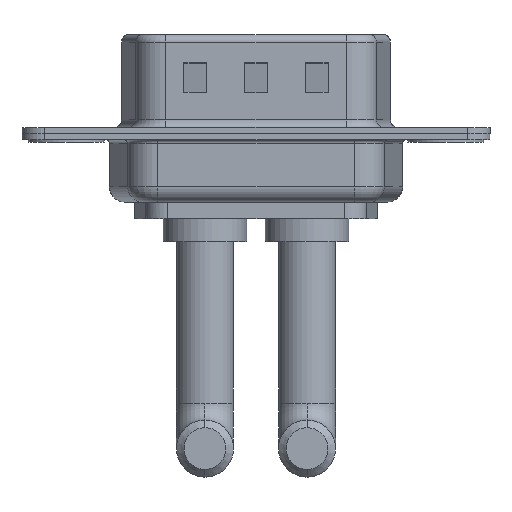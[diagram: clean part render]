
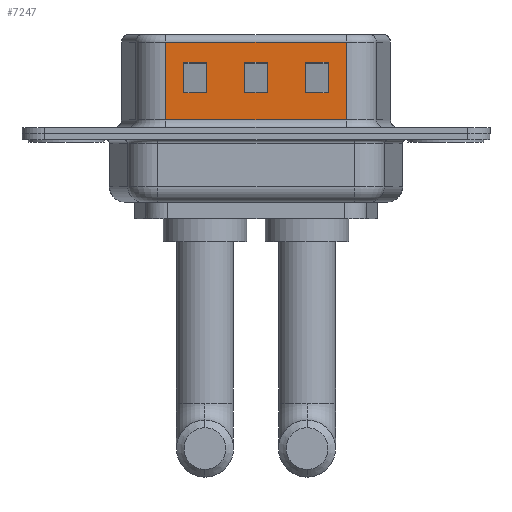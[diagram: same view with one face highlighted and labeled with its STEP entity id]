
A CAD part, front view. The second image highlights one B-rep face of the part: STEP entity #7247.
In plain terms, the highlighted planar face has unit normal (0, -1, 0).
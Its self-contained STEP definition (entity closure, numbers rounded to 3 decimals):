
#144 = CARTESIAN_POINT ( 'NONE',  ( 17.25, -4.55, 4.705 ) ) ;
#253 = VERTEX_POINT ( 'NONE', #11063 ) ;
#267 = VECTOR ( 'NONE', #5261, 1000. ) ;
#295 = EDGE_CURVE ( 'NONE', #964, #10683, #6149, .T. ) ;
#341 = DIRECTION ( 'NONE',  ( 0., 1., 0. ) ) ;
#506 = CARTESIAN_POINT ( 'NONE',  ( 6.549, -4.55, 6.52 ) ) ;
#653 = VECTOR ( 'NONE', #3412, 1000. ) ;
#688 = VECTOR ( 'NONE', #11170, 1000. ) ;
#964 = VERTEX_POINT ( 'NONE', #9049 ) ;
#1160 = EDGE_CURVE ( 'NONE', #10683, #10582, #6900, .T. ) ;
#1284 = DIRECTION ( 'NONE',  ( -1., 0., 0. ) ) ;
#1363 = CARTESIAN_POINT ( 'NONE',  ( 14.451, -4.55, 4.705 ) ) ;
#1442 = ORIENTED_EDGE ( 'NONE', *, *, #1997, .T. ) ;
#1643 = VECTOR ( 'NONE', #6165, 1000. ) ;
#1785 = CARTESIAN_POINT ( 'NONE',  ( 6.549, -4.55, 6.02 ) ) ;
#1997 = EDGE_CURVE ( 'NONE', #6853, #8826, #4202, .T. ) ;
#2039 = CARTESIAN_POINT ( 'NONE',  ( 13.25, -4.55, 2.705 ) ) ;
#2071 = EDGE_CURVE ( 'NONE', #9340, #253, #3422, .T. ) ;
#2237 = FACE_BOUND ( 'NONE', #9575, .T. ) ;
#2281 = EDGE_LOOP ( 'NONE', ( #9515, #8739, #8007, #7987 ) ) ;
#2312 = ORIENTED_EDGE ( 'NONE', *, *, #5085, .T. ) ;
#2397 = CARTESIAN_POINT ( 'NONE',  ( 9.25, -4.55, 6.52 ) ) ;
#2777 = VECTOR ( 'NONE', #11367, 1000. ) ;
#2842 = EDGE_CURVE ( 'NONE', #8517, #9124, #3017, .T. ) ;
#2870 = VECTOR ( 'NONE', #12316, 1000. ) ;
#3017 = LINE ( 'NONE', #1363, #4878 ) ;
#3307 = VECTOR ( 'NONE', #10962, 1000. ) ;
#3375 = VERTEX_POINT ( 'NONE', #144 ) ;
#3412 = DIRECTION ( 'NONE',  ( -1., 0., 0. ) ) ;
#3422 = LINE ( 'NONE', #7482, #2777 ) ;
#3617 = CARTESIAN_POINT ( 'NONE',  ( 13.25, -4.55, 4.705 ) ) ;
#3767 = ORIENTED_EDGE ( 'NONE', *, *, #3892, .T. ) ;
#3892 = EDGE_CURVE ( 'NONE', #3948, #8653, #11159, .T. ) ;
#3900 = LINE ( 'NONE', #7791, #11206 ) ;
#3910 = VECTOR ( 'NONE', #8266, 1000. ) ;
#3948 = VERTEX_POINT ( 'NONE', #9198 ) ;
#4017 = CARTESIAN_POINT ( 'NONE',  ( 17.25, -4.55, 6.52 ) ) ;
#4044 = DIRECTION ( 'NONE',  ( 0., 0., 1. ) ) ;
#4202 = LINE ( 'NONE', #6280, #1643 ) ;
#4217 = FACE_BOUND ( 'NONE', #6305, .T. ) ;
#4375 = ORIENTED_EDGE ( 'NONE', *, *, #2842, .T. ) ;
#4878 = VECTOR ( 'NONE', #10030, 1000. ) ;
#5085 = EDGE_CURVE ( 'NONE', #5225, #9340, #10999, .T. ) ;
#5095 = CARTESIAN_POINT ( 'NONE',  ( 18.451, -4.55, 2.705 ) ) ;
#5136 = DIRECTION ( 'NONE',  ( 0., 0., -1. ) ) ;
#5143 = VECTOR ( 'NONE', #4044, 1000. ) ;
#5175 = FACE_OUTER_BOUND ( 'NONE', #9629, .T. ) ;
#5225 = VERTEX_POINT ( 'NONE', #1785 ) ;
#5229 = DIRECTION ( 'NONE',  ( 0., 0., -1. ) ) ;
#5239 = ORIENTED_EDGE ( 'NONE', *, *, #6172, .T. ) ;
#5261 = DIRECTION ( 'NONE',  ( 0., 0., 1. ) ) ;
#5322 = CARTESIAN_POINT ( 'NONE',  ( 18.451, -4.55, 6.02 ) ) ;
#5388 = ORIENTED_EDGE ( 'NONE', *, *, #11726, .F. ) ;
#5398 = DIRECTION ( 'NONE',  ( 1., 0., 0. ) ) ;
#5462 = ORIENTED_EDGE ( 'NONE', *, *, #12061, .T. ) ;
#5811 = CARTESIAN_POINT ( 'NONE',  ( 9.25, -4.55, 4.705 ) ) ;
#5989 = LINE ( 'NONE', #4017, #10405 ) ;
#6106 = PLANE ( 'NONE',  #8422 ) ;
#6149 = LINE ( 'NONE', #7097, #653 ) ;
#6165 = DIRECTION ( 'NONE',  ( -1., 0., 0. ) ) ;
#6172 = EDGE_CURVE ( 'NONE', #12461, #10830, #7255, .T. ) ;
#6252 = LINE ( 'NONE', #12365, #10205 ) ;
#6280 = CARTESIAN_POINT ( 'NONE',  ( 14.451, -4.55, 2.705 ) ) ;
#6305 = EDGE_LOOP ( 'NONE', ( #3767, #5462, #5239, #12382 ) ) ;
#6853 = VERTEX_POINT ( 'NONE', #7168 ) ;
#6900 = LINE ( 'NONE', #9080, #5143 ) ;
#7043 = CARTESIAN_POINT ( 'NONE',  ( 11.75, -4.55, 2.705 ) ) ;
#7054 = EDGE_CURVE ( 'NONE', #9056, #5225, #7284, .T. ) ;
#7097 = CARTESIAN_POINT ( 'NONE',  ( 22.451, -4.55, 2.705 ) ) ;
#7168 = CARTESIAN_POINT ( 'NONE',  ( 9.25, -4.55, 2.705 ) ) ;
#7247 = ADVANCED_FACE ( 'NONE', ( #2237, #9059, #4217, #5175 ), #6106, .F. ) ;
#7255 = LINE ( 'NONE', #5095, #11838 ) ;
#7284 = LINE ( 'NONE', #5322, #688 ) ;
#7341 = ORIENTED_EDGE ( 'NONE', *, *, #12446, .T. ) ;
#7358 = CARTESIAN_POINT ( 'NONE',  ( 22.451, -4.55, 4.705 ) ) ;
#7482 = CARTESIAN_POINT ( 'NONE',  ( 18.451, -4.55, 0.9 ) ) ;
#7503 = VECTOR ( 'NONE', #5136, 1000. ) ;
#7791 = CARTESIAN_POINT ( 'NONE',  ( 11.75, -4.55, 6.52 ) ) ;
#7889 = LINE ( 'NONE', #11766, #267 ) ;
#7987 = ORIENTED_EDGE ( 'NONE', *, *, #11320, .T. ) ;
#8007 = ORIENTED_EDGE ( 'NONE', *, *, #1160, .T. ) ;
#8093 = CARTESIAN_POINT ( 'NONE',  ( 18.451, -4.55, 6.52 ) ) ;
#8266 = DIRECTION ( 'NONE',  ( 0., 0., -1. ) ) ;
#8272 = CARTESIAN_POINT ( 'NONE',  ( 15.75, -4.55, 4.705 ) ) ;
#8422 = AXIS2_PLACEMENT_3D ( 'NONE', #8093, #341, #11966 ) ;
#8429 = DIRECTION ( 'NONE',  ( 0., 0., -1. ) ) ;
#8430 = CARTESIAN_POINT ( 'NONE',  ( 18.451, -4.55, 4.705 ) ) ;
#8455 = CARTESIAN_POINT ( 'NONE',  ( 15.75, -4.55, 2.705 ) ) ;
#8517 = VERTEX_POINT ( 'NONE', #10324 ) ;
#8653 = VERTEX_POINT ( 'NONE', #3617 ) ;
#8739 = ORIENTED_EDGE ( 'NONE', *, *, #295, .T. ) ;
#8772 = ORIENTED_EDGE ( 'NONE', *, *, #8790, .T. ) ;
#8790 = EDGE_CURVE ( 'NONE', #9124, #6853, #10870, .T. ) ;
#8826 = VERTEX_POINT ( 'NONE', #11934 ) ;
#8997 = LINE ( 'NONE', #9837, #3307 ) ;
#9049 = CARTESIAN_POINT ( 'NONE',  ( 17.25, -4.55, 2.705 ) ) ;
#9056 = VERTEX_POINT ( 'NONE', #10480 ) ;
#9059 = FACE_BOUND ( 'NONE', #2281, .T. ) ;
#9080 = CARTESIAN_POINT ( 'NONE',  ( 15.75, -4.55, 6.52 ) ) ;
#9096 = CARTESIAN_POINT ( 'NONE',  ( 6.549, -4.55, 0.9 ) ) ;
#9124 = VERTEX_POINT ( 'NONE', #5811 ) ;
#9198 = CARTESIAN_POINT ( 'NONE',  ( 11.75, -4.55, 4.705 ) ) ;
#9340 = VERTEX_POINT ( 'NONE', #9096 ) ;
#9515 = ORIENTED_EDGE ( 'NONE', *, *, #9964, .T. ) ;
#9575 = EDGE_LOOP ( 'NONE', ( #8772, #1442, #7341, #4375 ) ) ;
#9629 = EDGE_LOOP ( 'NONE', ( #5388, #11716, #2312, #9682 ) ) ;
#9682 = ORIENTED_EDGE ( 'NONE', *, *, #2071, .T. ) ;
#9837 = CARTESIAN_POINT ( 'NONE',  ( 13.25, -4.55, 6.52 ) ) ;
#9964 = EDGE_CURVE ( 'NONE', #3375, #964, #5989, .T. ) ;
#10030 = DIRECTION ( 'NONE',  ( 1., 0., 0. ) ) ;
#10205 = VECTOR ( 'NONE', #8429, 1000. ) ;
#10324 = CARTESIAN_POINT ( 'NONE',  ( 7.75, -4.55, 4.705 ) ) ;
#10405 = VECTOR ( 'NONE', #5229, 1000. ) ;
#10480 = CARTESIAN_POINT ( 'NONE',  ( 18.451, -4.55, 6.02 ) ) ;
#10582 = VERTEX_POINT ( 'NONE', #8272 ) ;
#10584 = DIRECTION ( 'NONE',  ( 0., 0., 1. ) ) ;
#10683 = VERTEX_POINT ( 'NONE', #8455 ) ;
#10830 = VERTEX_POINT ( 'NONE', #7043 ) ;
#10870 = LINE ( 'NONE', #2397, #7503 ) ;
#10962 = DIRECTION ( 'NONE',  ( 0., 0., -1. ) ) ;
#10999 = LINE ( 'NONE', #506, #3910 ) ;
#11063 = CARTESIAN_POINT ( 'NONE',  ( 18.451, -4.55, 0.9 ) ) ;
#11159 = LINE ( 'NONE', #8430, #2870 ) ;
#11170 = DIRECTION ( 'NONE',  ( -1., 0., 0. ) ) ;
#11206 = VECTOR ( 'NONE', #10584, 1000. ) ;
#11228 = VECTOR ( 'NONE', #5398, 1000. ) ;
#11320 = EDGE_CURVE ( 'NONE', #10582, #3375, #12197, .T. ) ;
#11367 = DIRECTION ( 'NONE',  ( 1., 0., 0. ) ) ;
#11716 = ORIENTED_EDGE ( 'NONE', *, *, #7054, .T. ) ;
#11726 = EDGE_CURVE ( 'NONE', #9056, #253, #6252, .T. ) ;
#11766 = CARTESIAN_POINT ( 'NONE',  ( 7.75, -4.55, 6.52 ) ) ;
#11838 = VECTOR ( 'NONE', #1284, 1000. ) ;
#11860 = EDGE_CURVE ( 'NONE', #10830, #3948, #3900, .T. ) ;
#11934 = CARTESIAN_POINT ( 'NONE',  ( 7.75, -4.55, 2.705 ) ) ;
#11966 = DIRECTION ( 'NONE',  ( -1., 0., 0. ) ) ;
#12061 = EDGE_CURVE ( 'NONE', #8653, #12461, #8997, .T. ) ;
#12197 = LINE ( 'NONE', #7358, #11228 ) ;
#12316 = DIRECTION ( 'NONE',  ( 1., 0., 0. ) ) ;
#12365 = CARTESIAN_POINT ( 'NONE',  ( 18.451, -4.55, 6.52 ) ) ;
#12382 = ORIENTED_EDGE ( 'NONE', *, *, #11860, .T. ) ;
#12446 = EDGE_CURVE ( 'NONE', #8826, #8517, #7889, .T. ) ;
#12461 = VERTEX_POINT ( 'NONE', #2039 ) ;
